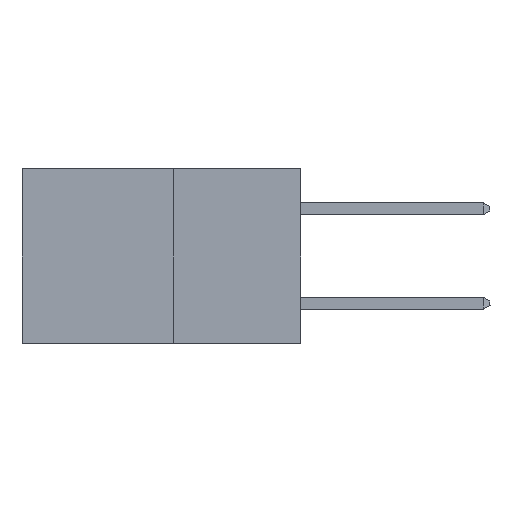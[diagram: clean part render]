
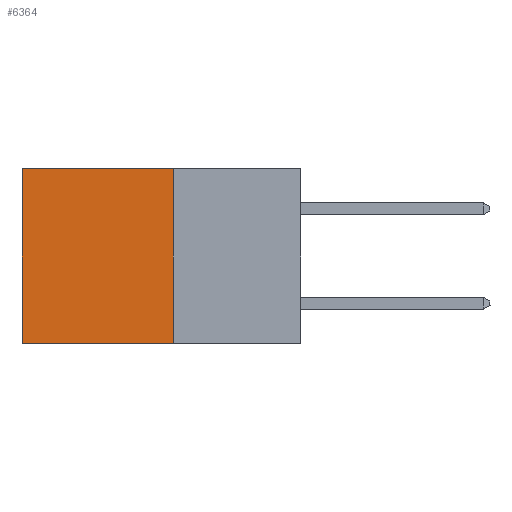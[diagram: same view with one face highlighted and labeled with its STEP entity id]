
A CAD part, left-side view. The second image highlights one B-rep face of the part: STEP entity #6364.
In plain terms, the highlighted planar face has unit normal (-1, 0, 0).
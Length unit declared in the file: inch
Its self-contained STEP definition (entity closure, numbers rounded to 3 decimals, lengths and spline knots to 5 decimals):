
#2361 = ORIENTED_EDGE ( 'NONE', *, *, #19497, .T. ) ;
#2726 = CARTESIAN_POINT ( 'NONE',  ( 0.277, 0.59, -0.37 ) ) ;
#2827 = CARTESIAN_POINT ( 'NONE',  ( 0.277, 0.59, 0. ) ) ;
#3034 = LINE ( 'NONE', #17917, #15827 ) ;
#3096 = ORIENTED_EDGE ( 'NONE', *, *, #7904, .F. ) ;
#3378 = ORIENTED_EDGE ( 'NONE', *, *, #10247, .T. ) ;
#4189 = EDGE_LOOP ( 'NONE', ( #2361, #15878, #3096, #3378 ) ) ;
#5476 = LINE ( 'NONE', #7553, #14302 ) ;
#5782 = VERTEX_POINT ( 'NONE', #5809 ) ;
#5809 = CARTESIAN_POINT ( 'NONE',  ( 0.277, 0.27, -0.37 ) ) ;
#5853 = VECTOR ( 'NONE', #16263, 39.37008 ) ;
#6364 = ADVANCED_FACE ( 'NONE', ( #9743 ), #13345, .F. ) ;
#6644 = VERTEX_POINT ( 'NONE', #9148 ) ;
#7360 = DIRECTION ( 'NONE',  ( 0., 0., -1. ) ) ;
#7553 = CARTESIAN_POINT ( 'NONE',  ( 0.277, 0.27, -0.37 ) ) ;
#7778 = DIRECTION ( 'NONE',  ( 0., 1., 0. ) ) ;
#7904 = EDGE_CURVE ( 'NONE', #6644, #5782, #5476, .T. ) ;
#7951 = CARTESIAN_POINT ( 'NONE',  ( 0.277, 0.27, 0. ) ) ;
#9148 = CARTESIAN_POINT ( 'NONE',  ( 0.277, 0.27, 0. ) ) ;
#9193 = EDGE_CURVE ( 'NONE', #5782, #16809, #3034, .T. ) ;
#9409 = AXIS2_PLACEMENT_3D ( 'NONE', #13204, #13177, #13157 ) ;
#9743 = FACE_OUTER_BOUND ( 'NONE', #4189, .T. ) ;
#10247 = EDGE_CURVE ( 'NONE', #6644, #14187, #17581, .T. ) ;
#13157 = DIRECTION ( 'NONE',  ( 0., 0., -1. ) ) ;
#13161 = VECTOR ( 'NONE', #7778, 39.37008 ) ;
#13177 = DIRECTION ( 'NONE',  ( 1., 0., 0. ) ) ;
#13204 = CARTESIAN_POINT ( 'NONE',  ( 0.277, 0.27, -0.37 ) ) ;
#13345 = PLANE ( 'NONE',  #9409 ) ;
#14187 = VERTEX_POINT ( 'NONE', #2827 ) ;
#14302 = VECTOR ( 'NONE', #7360, 39.37008 ) ;
#14587 = CARTESIAN_POINT ( 'NONE',  ( 0.277, 0.59, -0.37 ) ) ;
#15195 = LINE ( 'NONE', #14587, #5853 ) ;
#15827 = VECTOR ( 'NONE', #17629, 39.37008 ) ;
#15878 = ORIENTED_EDGE ( 'NONE', *, *, #9193, .F. ) ;
#16263 = DIRECTION ( 'NONE',  ( 0., 0., -1. ) ) ;
#16809 = VERTEX_POINT ( 'NONE', #2726 ) ;
#17581 = LINE ( 'NONE', #7951, #13161 ) ;
#17629 = DIRECTION ( 'NONE',  ( 0., 1., 0. ) ) ;
#17917 = CARTESIAN_POINT ( 'NONE',  ( 0.277, 0.27, -0.37 ) ) ;
#19497 = EDGE_CURVE ( 'NONE', #14187, #16809, #15195, .T. ) ;
